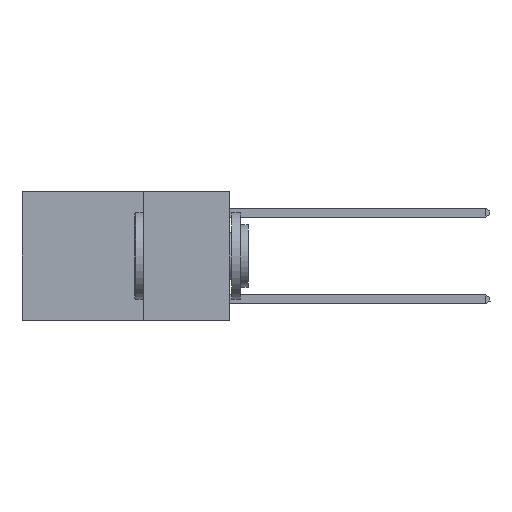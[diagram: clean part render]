
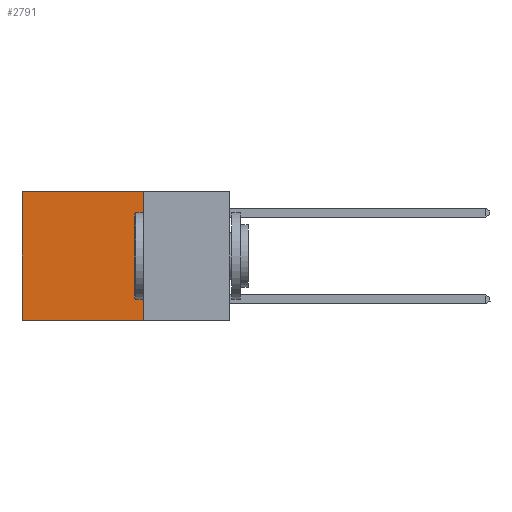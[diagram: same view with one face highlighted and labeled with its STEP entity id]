
A CAD part, left-side view. The second image highlights one B-rep face of the part: STEP entity #2791.
In plain terms, the highlighted planar face has unit normal (-1, 0, 0).
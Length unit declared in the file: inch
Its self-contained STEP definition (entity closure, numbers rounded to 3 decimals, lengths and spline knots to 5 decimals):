
#484 = ORIENTED_EDGE ( 'NONE', *, *, #24811, .T. ) ;
#1487 = VECTOR ( 'NONE', #26359, 39.37008 ) ;
#2791 = ADVANCED_FACE ( 'NONE', ( #4452 ), #24495, .F. ) ;
#3630 = DIRECTION ( 'NONE',  ( 0., 0., -1. ) ) ;
#3663 = ORIENTED_EDGE ( 'NONE', *, *, #26143, .T. ) ;
#4452 = FACE_OUTER_BOUND ( 'NONE', #11079, .T. ) ;
#5045 = VECTOR ( 'NONE', #24159, 39.37008 ) ;
#5813 = CARTESIAN_POINT ( 'NONE',  ( 0.2625, 0.6, 0. ) ) ;
#5836 = CARTESIAN_POINT ( 'NONE',  ( 0.2625, 0.6, 0. ) ) ;
#7535 = LINE ( 'NONE', #24263, #1487 ) ;
#8254 = CARTESIAN_POINT ( 'NONE',  ( 0.2625, 0.25, 0. ) ) ;
#9583 = CARTESIAN_POINT ( 'NONE',  ( 0.2625, 0.25, -0.37 ) ) ;
#9668 = VECTOR ( 'NONE', #24605, 39.37008 ) ;
#10328 = LINE ( 'NONE', #22074, #5045 ) ;
#11079 = EDGE_LOOP ( 'NONE', ( #3663, #27360, #16871, #484 ) ) ;
#11299 = AXIS2_PLACEMENT_3D ( 'NONE', #13987, #24584, #11809 ) ;
#11809 = DIRECTION ( 'NONE',  ( 0., 0., -1. ) ) ;
#13987 = CARTESIAN_POINT ( 'NONE',  ( 0.2625, 0.25, 0. ) ) ;
#14538 = LINE ( 'NONE', #5813, #20182 ) ;
#14713 = VERTEX_POINT ( 'NONE', #25354 ) ;
#16586 = VERTEX_POINT ( 'NONE', #8254 ) ;
#16871 = ORIENTED_EDGE ( 'NONE', *, *, #17624, .F. ) ;
#17624 = EDGE_CURVE ( 'NONE', #16586, #18578, #10328, .T. ) ;
#17971 = VERTEX_POINT ( 'NONE', #5836 ) ;
#18578 = VERTEX_POINT ( 'NONE', #9583 ) ;
#20182 = VECTOR ( 'NONE', #3630, 39.37008 ) ;
#22074 = CARTESIAN_POINT ( 'NONE',  ( 0.2625, 0.25, 0. ) ) ;
#22518 = CARTESIAN_POINT ( 'NONE',  ( 0.2625, 0.25, -0.37 ) ) ;
#24159 = DIRECTION ( 'NONE',  ( 0., 0., -1. ) ) ;
#24263 = CARTESIAN_POINT ( 'NONE',  ( 0.2625, 0.25, 0. ) ) ;
#24495 = PLANE ( 'NONE',  #11299 ) ;
#24584 = DIRECTION ( 'NONE',  ( 1., 0., 0. ) ) ;
#24605 = DIRECTION ( 'NONE',  ( 0., 1., 0. ) ) ;
#24811 = EDGE_CURVE ( 'NONE', #16586, #17971, #7535, .T. ) ;
#25354 = CARTESIAN_POINT ( 'NONE',  ( 0.2625, 0.6, -0.37 ) ) ;
#25821 = EDGE_CURVE ( 'NONE', #18578, #14713, #26721, .T. ) ;
#26143 = EDGE_CURVE ( 'NONE', #17971, #14713, #14538, .T. ) ;
#26359 = DIRECTION ( 'NONE',  ( 0., 1., 0. ) ) ;
#26721 = LINE ( 'NONE', #22518, #9668 ) ;
#27360 = ORIENTED_EDGE ( 'NONE', *, *, #25821, .F. ) ;
